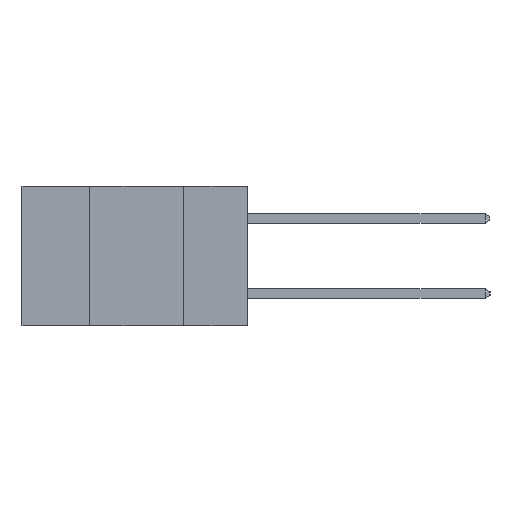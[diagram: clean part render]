
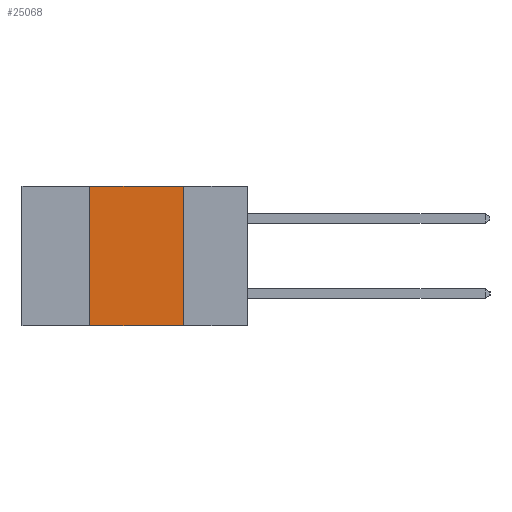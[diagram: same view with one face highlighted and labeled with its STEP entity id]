
A CAD part, left-side view. The second image highlights one B-rep face of the part: STEP entity #25068.
In plain terms, the highlighted planar face has unit normal (-1, 0, 0).
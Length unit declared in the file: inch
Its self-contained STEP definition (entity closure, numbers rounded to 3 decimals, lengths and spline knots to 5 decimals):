
#240 = FACE_OUTER_BOUND ( 'NONE', #15484, .T. ) ;
#1386 = LINE ( 'NONE', #4444, #21927 ) ;
#1528 = CARTESIAN_POINT ( 'NONE',  ( 0., 0.17, 0. ) ) ;
#1760 = EDGE_CURVE ( 'NONE', #2018, #12204, #5801, .T. ) ;
#2018 = VERTEX_POINT ( 'NONE', #1528 ) ;
#2349 = AXIS2_PLACEMENT_3D ( 'NONE', #9294, #11308, #25021 ) ;
#2519 = LINE ( 'NONE', #20575, #13168 ) ;
#3820 = EDGE_CURVE ( 'NONE', #9096, #2018, #2519, .T. ) ;
#4444 = CARTESIAN_POINT ( 'NONE',  ( 0., 0.42, -0.37 ) ) ;
#5157 = ORIENTED_EDGE ( 'NONE', *, *, #7320, .F. ) ;
#5590 = CARTESIAN_POINT ( 'NONE',  ( 0., 0.42, -0.37 ) ) ;
#5677 = DIRECTION ( 'NONE',  ( 0., -1., 0. ) ) ;
#5801 = LINE ( 'NONE', #18861, #21014 ) ;
#6016 = LINE ( 'NONE', #15604, #20610 ) ;
#7286 = PLANE ( 'NONE',  #2349 ) ;
#7320 = EDGE_CURVE ( 'NONE', #12256, #9096, #1386, .T. ) ;
#7722 = ORIENTED_EDGE ( 'NONE', *, *, #1760, .F. ) ;
#9096 = VERTEX_POINT ( 'NONE', #23689 ) ;
#9294 = CARTESIAN_POINT ( 'NONE',  ( 0., 0.6, 0. ) ) ;
#11308 = DIRECTION ( 'NONE',  ( 1., 0., 0. ) ) ;
#12204 = VERTEX_POINT ( 'NONE', #17348 ) ;
#12256 = VERTEX_POINT ( 'NONE', #5590 ) ;
#13168 = VECTOR ( 'NONE', #21951, 39.37008 ) ;
#13860 = ORIENTED_EDGE ( 'NONE', *, *, #23073, .T. ) ;
#15484 = EDGE_LOOP ( 'NONE', ( #7722, #20860, #5157, #13860 ) ) ;
#15604 = CARTESIAN_POINT ( 'NONE',  ( 0., 0.6, -0.37 ) ) ;
#17348 = CARTESIAN_POINT ( 'NONE',  ( 0., 0.17, -0.37 ) ) ;
#18861 = CARTESIAN_POINT ( 'NONE',  ( 0., 0.17, -0.37 ) ) ;
#18950 = DIRECTION ( 'NONE',  ( 0., 0., -1. ) ) ;
#20575 = CARTESIAN_POINT ( 'NONE',  ( 0., 0.6, 0. ) ) ;
#20610 = VECTOR ( 'NONE', #5677, 39.37008 ) ;
#20860 = ORIENTED_EDGE ( 'NONE', *, *, #3820, .F. ) ;
#21014 = VECTOR ( 'NONE', #18950, 39.37008 ) ;
#21927 = VECTOR ( 'NONE', #22302, 39.37008 ) ;
#21951 = DIRECTION ( 'NONE',  ( 0., -1., 0. ) ) ;
#22302 = DIRECTION ( 'NONE',  ( 0., 0., 1. ) ) ;
#23073 = EDGE_CURVE ( 'NONE', #12256, #12204, #6016, .T. ) ;
#23689 = CARTESIAN_POINT ( 'NONE',  ( 0., 0.42, 0. ) ) ;
#25021 = DIRECTION ( 'NONE',  ( 0., 0., -1. ) ) ;
#25068 = ADVANCED_FACE ( 'NONE', ( #240 ), #7286, .F. ) ;
